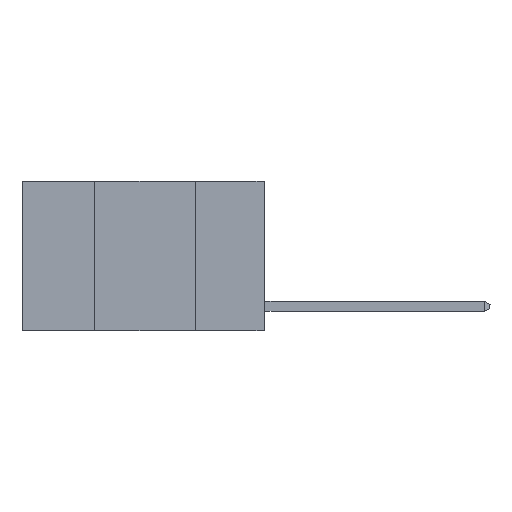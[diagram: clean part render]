
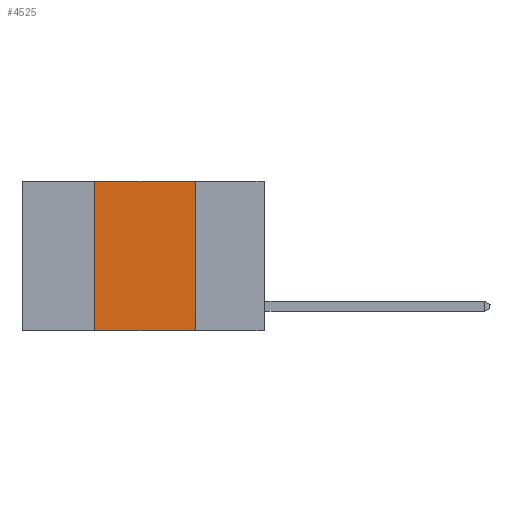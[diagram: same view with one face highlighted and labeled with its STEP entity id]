
A CAD part, left-side view. The second image highlights one B-rep face of the part: STEP entity #4525.
In plain terms, the highlighted planar face has unit normal (-1, 0, 0).
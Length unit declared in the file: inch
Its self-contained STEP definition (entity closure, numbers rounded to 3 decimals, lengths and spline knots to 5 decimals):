
#4195 = CARTESIAN_POINT ( 'NONE',  ( 0., 0.17, 0. ) ) ;
#4525 = ADVANCED_FACE ( 'NONE', ( #15095 ), #21664, .F. ) ;
#6087 = DIRECTION ( 'NONE',  ( 0., 0., -1. ) ) ;
#6602 = DIRECTION ( 'NONE',  ( 0., -1., 0. ) ) ;
#7488 = EDGE_CURVE ( 'NONE', #24540, #24877, #7649, .T. ) ;
#7649 = LINE ( 'NONE', #26457, #20111 ) ;
#8267 = CARTESIAN_POINT ( 'NONE',  ( 0., 0.17, 0. ) ) ;
#8432 = CARTESIAN_POINT ( 'NONE',  ( 0., 0.6, 0. ) ) ;
#8725 = CARTESIAN_POINT ( 'NONE',  ( 0., 0.6, 0. ) ) ;
#8976 = LINE ( 'NONE', #8725, #19362 ) ;
#9147 = CARTESIAN_POINT ( 'NONE',  ( 0., 0.17, -0.37 ) ) ;
#10315 = EDGE_CURVE ( 'NONE', #24540, #10415, #11291, .T. ) ;
#10415 = VERTEX_POINT ( 'NONE', #9147 ) ;
#11291 = LINE ( 'NONE', #28162, #25814 ) ;
#11397 = VERTEX_POINT ( 'NONE', #4195 ) ;
#11677 = ORIENTED_EDGE ( 'NONE', *, *, #10315, .T. ) ;
#12786 = ORIENTED_EDGE ( 'NONE', *, *, #13849, .F. ) ;
#13849 = EDGE_CURVE ( 'NONE', #24877, #11397, #8976, .T. ) ;
#13951 = CARTESIAN_POINT ( 'NONE',  ( 0., 0.42, -0.37 ) ) ;
#15095 = FACE_OUTER_BOUND ( 'NONE', #28079, .T. ) ;
#16360 = CARTESIAN_POINT ( 'NONE',  ( 0., 0.42, 0. ) ) ;
#16614 = ORIENTED_EDGE ( 'NONE', *, *, #18007, .F. ) ;
#16674 = LINE ( 'NONE', #8267, #20141 ) ;
#18007 = EDGE_CURVE ( 'NONE', #11397, #10415, #16674, .T. ) ;
#18085 = ORIENTED_EDGE ( 'NONE', *, *, #7488, .F. ) ;
#18313 = DIRECTION ( 'NONE',  ( 0., 0., 1. ) ) ;
#19362 = VECTOR ( 'NONE', #20480, 39.37008 ) ;
#20111 = VECTOR ( 'NONE', #18313, 39.37008 ) ;
#20141 = VECTOR ( 'NONE', #28164, 39.37008 ) ;
#20480 = DIRECTION ( 'NONE',  ( 0., -1., 0. ) ) ;
#21664 = PLANE ( 'NONE',  #28063 ) ;
#23883 = DIRECTION ( 'NONE',  ( 1., 0., 0. ) ) ;
#24540 = VERTEX_POINT ( 'NONE', #13951 ) ;
#24877 = VERTEX_POINT ( 'NONE', #16360 ) ;
#25814 = VECTOR ( 'NONE', #6602, 39.37008 ) ;
#26457 = CARTESIAN_POINT ( 'NONE',  ( 0., 0.42, 0. ) ) ;
#28063 = AXIS2_PLACEMENT_3D ( 'NONE', #8432, #23883, #6087 ) ;
#28079 = EDGE_LOOP ( 'NONE', ( #16614, #12786, #18085, #11677 ) ) ;
#28162 = CARTESIAN_POINT ( 'NONE',  ( 0., 0.6, -0.37 ) ) ;
#28164 = DIRECTION ( 'NONE',  ( 0., 0., -1. ) ) ;
